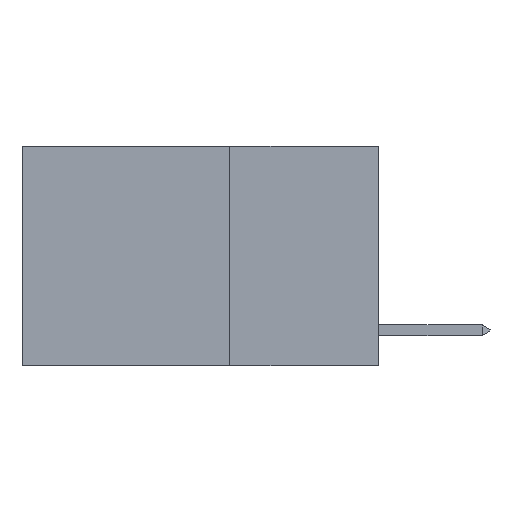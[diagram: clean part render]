
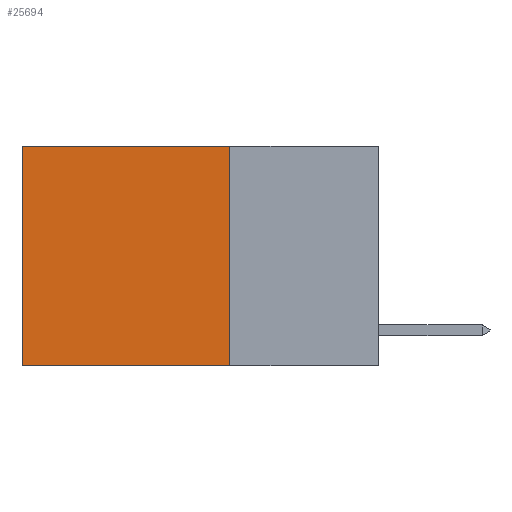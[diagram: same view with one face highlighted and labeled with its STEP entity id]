
A CAD part, left-side view. The second image highlights one B-rep face of the part: STEP entity #25694.
In plain terms, the highlighted planar face has unit normal (-1, 0, 0).
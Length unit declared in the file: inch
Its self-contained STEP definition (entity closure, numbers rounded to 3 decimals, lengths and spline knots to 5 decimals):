
#174 = DIRECTION ( 'NONE',  ( 0., 0., -1. ) ) ;
#668 = CARTESIAN_POINT ( 'NONE',  ( 0.2625, 0.25, 0. ) ) ;
#1310 = CARTESIAN_POINT ( 'NONE',  ( 0.2625, 0.25, 0. ) ) ;
#1425 = VECTOR ( 'NONE', #10514, 39.37008 ) ;
#2981 = DIRECTION ( 'NONE',  ( 0., 0., -1. ) ) ;
#4609 = VECTOR ( 'NONE', #174, 39.37008 ) ;
#6674 = PLANE ( 'NONE',  #25832 ) ;
#8588 = CARTESIAN_POINT ( 'NONE',  ( 0.2625, 0.6, 0. ) ) ;
#10514 = DIRECTION ( 'NONE',  ( 0., 1., 0. ) ) ;
#10736 = LINE ( 'NONE', #8588, #18961 ) ;
#11402 = CARTESIAN_POINT ( 'NONE',  ( 0.2625, 0.25, -0.37 ) ) ;
#11459 = VERTEX_POINT ( 'NONE', #26024 ) ;
#11543 = EDGE_CURVE ( 'NONE', #25283, #22130, #18483, .T. ) ;
#12375 = CARTESIAN_POINT ( 'NONE',  ( 0.2625, 0.25, -0.37 ) ) ;
#13867 = ORIENTED_EDGE ( 'NONE', *, *, #11543, .F. ) ;
#14611 = FACE_OUTER_BOUND ( 'NONE', #16709, .T. ) ;
#14898 = DIRECTION ( 'NONE',  ( 0., 0., -1. ) ) ;
#14902 = CARTESIAN_POINT ( 'NONE',  ( 0.2625, 0.25, 0. ) ) ;
#16709 = EDGE_LOOP ( 'NONE', ( #19149, #25490, #13867, #20423 ) ) ;
#18483 = LINE ( 'NONE', #668, #4609 ) ;
#18961 = VECTOR ( 'NONE', #14898, 39.37008 ) ;
#19149 = ORIENTED_EDGE ( 'NONE', *, *, #23876, .T. ) ;
#19544 = VERTEX_POINT ( 'NONE', #20162 ) ;
#20162 = CARTESIAN_POINT ( 'NONE',  ( 0.2625, 0.6, -0.37 ) ) ;
#20423 = ORIENTED_EDGE ( 'NONE', *, *, #23707, .T. ) ;
#21096 = LINE ( 'NONE', #1310, #25044 ) ;
#21680 = CARTESIAN_POINT ( 'NONE',  ( 0.2625, 0.25, 0. ) ) ;
#22130 = VERTEX_POINT ( 'NONE', #12375 ) ;
#23321 = DIRECTION ( 'NONE',  ( 1., 0., 0. ) ) ;
#23707 = EDGE_CURVE ( 'NONE', #25283, #11459, #21096, .T. ) ;
#23876 = EDGE_CURVE ( 'NONE', #11459, #19544, #10736, .T. ) ;
#24483 = LINE ( 'NONE', #11402, #1425 ) ;
#25044 = VECTOR ( 'NONE', #25943, 39.37008 ) ;
#25283 = VERTEX_POINT ( 'NONE', #14902 ) ;
#25490 = ORIENTED_EDGE ( 'NONE', *, *, #26526, .F. ) ;
#25694 = ADVANCED_FACE ( 'NONE', ( #14611 ), #6674, .F. ) ;
#25832 = AXIS2_PLACEMENT_3D ( 'NONE', #21680, #23321, #2981 ) ;
#25943 = DIRECTION ( 'NONE',  ( 0., 1., 0. ) ) ;
#26024 = CARTESIAN_POINT ( 'NONE',  ( 0.2625, 0.6, 0. ) ) ;
#26526 = EDGE_CURVE ( 'NONE', #22130, #19544, #24483, .T. ) ;
